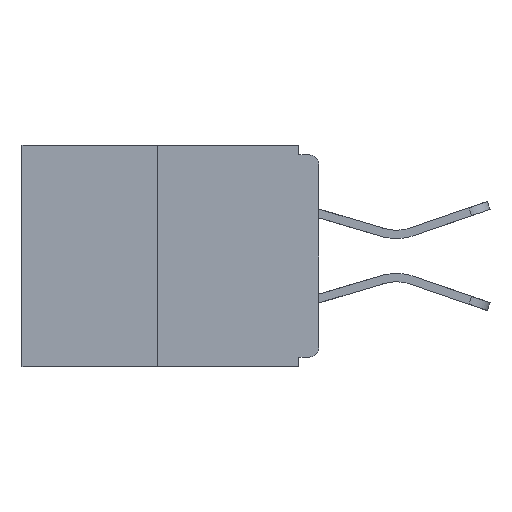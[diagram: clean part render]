
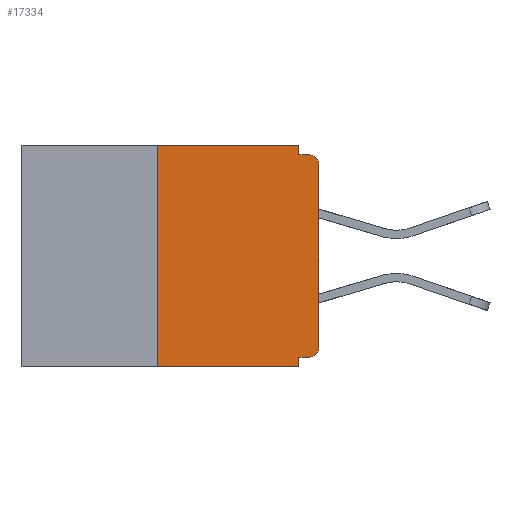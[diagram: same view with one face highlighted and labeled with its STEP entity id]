
A CAD part, left-side view. The second image highlights one B-rep face of the part: STEP entity #17334.
In plain terms, the highlighted planar face has unit normal (-1, 0, 0).
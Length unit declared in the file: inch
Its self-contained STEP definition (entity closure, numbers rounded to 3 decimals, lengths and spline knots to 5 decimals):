
#476 = DIRECTION ( 'NONE',  ( 0., -1., 0. ) ) ;
#604 = VERTEX_POINT ( 'NONE', #11326 ) ;
#811 = AXIS2_PLACEMENT_3D ( 'NONE', #4466, #8311, #21504 ) ;
#1052 = VERTEX_POINT ( 'NONE', #16371 ) ;
#1828 = LINE ( 'NONE', #9717, #11923 ) ;
#2422 = EDGE_CURVE ( 'NONE', #1052, #11686, #14587, .T. ) ;
#3073 = ORIENTED_EDGE ( 'NONE', *, *, #19672, .F. ) ;
#3425 = CARTESIAN_POINT ( 'NONE',  ( 0., 0.46, 0. ) ) ;
#3484 = DIRECTION ( 'NONE',  ( 0., 1., 0. ) ) ;
#3548 = LINE ( 'NONE', #11726, #23064 ) ;
#3760 = VERTEX_POINT ( 'NONE', #22604 ) ;
#4360 = EDGE_CURVE ( 'NONE', #604, #9836, #22771, .T. ) ;
#4434 = CARTESIAN_POINT ( 'NONE',  ( 0., 0.031, -0.328 ) ) ;
#4466 = CARTESIAN_POINT ( 'NONE',  ( 0., 0.015, -0.313 ) ) ;
#4474 = CARTESIAN_POINT ( 'NONE',  ( 0., 0.031, -0.343 ) ) ;
#5195 = ORIENTED_EDGE ( 'NONE', *, *, #11284, .F. ) ;
#5347 = DIRECTION ( 'NONE',  ( 0., 0., 1. ) ) ;
#5364 = CARTESIAN_POINT ( 'NONE',  ( 0., 0.031, 0. ) ) ;
#6048 = FACE_OUTER_BOUND ( 'NONE', #15055, .T. ) ;
#6480 = CARTESIAN_POINT ( 'NONE',  ( 0., 0.25, -0.343 ) ) ;
#6484 = VECTOR ( 'NONE', #22946, 39.37008 ) ;
#7331 = EDGE_CURVE ( 'NONE', #22307, #22441, #24428, .T. ) ;
#7504 = DIRECTION ( 'NONE',  ( 0., 0., -1. ) ) ;
#7550 = ORIENTED_EDGE ( 'NONE', *, *, #15172, .F. ) ;
#7630 = CARTESIAN_POINT ( 'NONE',  ( 0., 0.015, -0.03 ) ) ;
#7817 = DIRECTION ( 'NONE',  ( 0., -1., 0. ) ) ;
#8311 = DIRECTION ( 'NONE',  ( -1., 0., 0. ) ) ;
#8402 = AXIS2_PLACEMENT_3D ( 'NONE', #7630, #11429, #19104 ) ;
#8534 = VERTEX_POINT ( 'NONE', #4474 ) ;
#8796 = LINE ( 'NONE', #22509, #12041 ) ;
#8813 = VERTEX_POINT ( 'NONE', #23105 ) ;
#8905 = ORIENTED_EDGE ( 'NONE', *, *, #7331, .F. ) ;
#9161 = CARTESIAN_POINT ( 'NONE',  ( 0., 0., 0. ) ) ;
#9643 = ORIENTED_EDGE ( 'NONE', *, *, #22589, .T. ) ;
#9672 = VECTOR ( 'NONE', #7817, 39.37008 ) ;
#9717 = CARTESIAN_POINT ( 'NONE',  ( 0., 0.031, 0. ) ) ;
#9836 = VERTEX_POINT ( 'NONE', #21317 ) ;
#10528 = LINE ( 'NONE', #22559, #9672 ) ;
#11284 = EDGE_CURVE ( 'NONE', #21359, #3760, #1828, .T. ) ;
#11326 = CARTESIAN_POINT ( 'NONE',  ( 0., 0., -0.03 ) ) ;
#11429 = DIRECTION ( 'NONE',  ( -1., 0., 0. ) ) ;
#11431 = DIRECTION ( 'NONE',  ( 0., 0., -1. ) ) ;
#11686 = VERTEX_POINT ( 'NONE', #4434 ) ;
#11726 = CARTESIAN_POINT ( 'NONE',  ( 0., 0.46, -0.343 ) ) ;
#11923 = VECTOR ( 'NONE', #15219, 39.37008 ) ;
#12041 = VECTOR ( 'NONE', #7504, 39.37008 ) ;
#12550 = CARTESIAN_POINT ( 'NONE',  ( 0., 0.25, 0. ) ) ;
#14434 = LINE ( 'NONE', #3425, #15627 ) ;
#14587 = LINE ( 'NONE', #22251, #20530 ) ;
#15055 = EDGE_LOOP ( 'NONE', ( #3073, #8905, #9643, #7550, #16326, #17207, #16896, #18938, #19124, #5195 ) ) ;
#15113 = CARTESIAN_POINT ( 'NONE',  ( 0., 0.46, 0. ) ) ;
#15172 = EDGE_CURVE ( 'NONE', #11686, #8534, #8796, .T. ) ;
#15219 = DIRECTION ( 'NONE',  ( 0., 0., -1. ) ) ;
#15450 = LINE ( 'NONE', #9161, #18395 ) ;
#15627 = VECTOR ( 'NONE', #22600, 39.37008 ) ;
#15787 = EDGE_CURVE ( 'NONE', #3760, #9836, #10528, .T. ) ;
#16049 = EDGE_CURVE ( 'NONE', #1052, #8813, #24029, .T. ) ;
#16326 = ORIENTED_EDGE ( 'NONE', *, *, #2422, .F. ) ;
#16371 = CARTESIAN_POINT ( 'NONE',  ( 0., 0.015, -0.328 ) ) ;
#16896 = ORIENTED_EDGE ( 'NONE', *, *, #19645, .T. ) ;
#17207 = ORIENTED_EDGE ( 'NONE', *, *, #16049, .T. ) ;
#17334 = ADVANCED_FACE ( 'NONE', ( #6048 ), #18863, .F. ) ;
#18395 = VECTOR ( 'NONE', #5347, 39.37008 ) ;
#18863 = PLANE ( 'NONE',  #24073 ) ;
#18938 = ORIENTED_EDGE ( 'NONE', *, *, #4360, .T. ) ;
#18942 = DIRECTION ( 'NONE',  ( 1., 0., 0. ) ) ;
#19104 = DIRECTION ( 'NONE',  ( 0., 0., -1. ) ) ;
#19124 = ORIENTED_EDGE ( 'NONE', *, *, #15787, .F. ) ;
#19645 = EDGE_CURVE ( 'NONE', #8813, #604, #15450, .T. ) ;
#19672 = EDGE_CURVE ( 'NONE', #22441, #21359, #14434, .T. ) ;
#20530 = VECTOR ( 'NONE', #3484, 39.37008 ) ;
#21156 = CARTESIAN_POINT ( 'NONE',  ( 0., 0.25, 0. ) ) ;
#21317 = CARTESIAN_POINT ( 'NONE',  ( 0., 0.015, -0.015 ) ) ;
#21359 = VERTEX_POINT ( 'NONE', #5364 ) ;
#21504 = DIRECTION ( 'NONE',  ( 0., 0., -1. ) ) ;
#22251 = CARTESIAN_POINT ( 'NONE',  ( 0., 0., -0.328 ) ) ;
#22307 = VERTEX_POINT ( 'NONE', #6480 ) ;
#22441 = VERTEX_POINT ( 'NONE', #12550 ) ;
#22509 = CARTESIAN_POINT ( 'NONE',  ( 0., 0.031, -0.343 ) ) ;
#22559 = CARTESIAN_POINT ( 'NONE',  ( 0., 0., -0.015 ) ) ;
#22589 = EDGE_CURVE ( 'NONE', #22307, #8534, #3548, .T. ) ;
#22600 = DIRECTION ( 'NONE',  ( 0., -1., 0. ) ) ;
#22604 = CARTESIAN_POINT ( 'NONE',  ( 0., 0.031, -0.015 ) ) ;
#22771 = CIRCLE ( 'NONE', #8402, 0.015 ) ;
#22946 = DIRECTION ( 'NONE',  ( 0., 0., 1. ) ) ;
#23064 = VECTOR ( 'NONE', #476, 39.37008 ) ;
#23105 = CARTESIAN_POINT ( 'NONE',  ( 0., 0., -0.313 ) ) ;
#24029 = CIRCLE ( 'NONE', #811, 0.015 ) ;
#24073 = AXIS2_PLACEMENT_3D ( 'NONE', #15113, #18942, #11431 ) ;
#24428 = LINE ( 'NONE', #21156, #6484 ) ;
